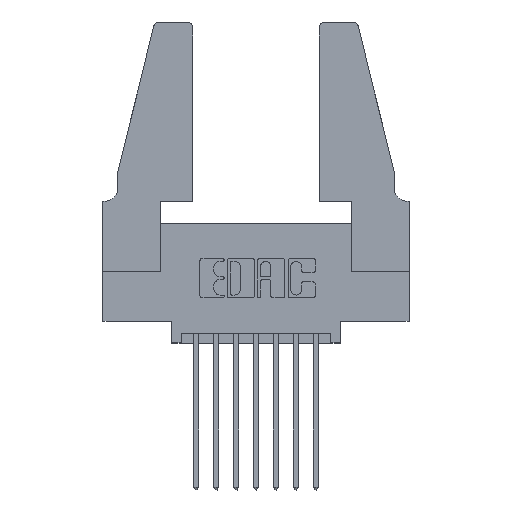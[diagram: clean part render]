
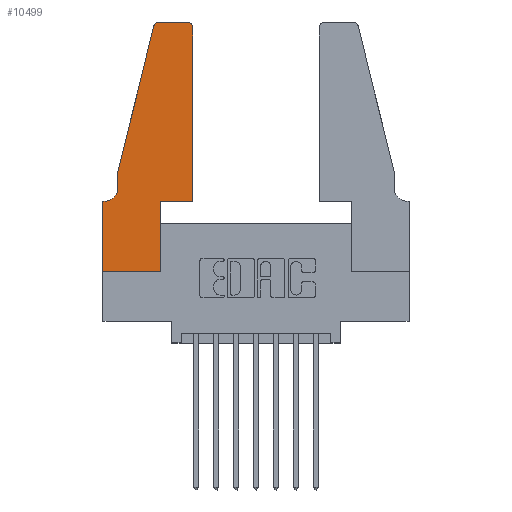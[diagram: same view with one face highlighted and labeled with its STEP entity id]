
A CAD part, top view. The second image highlights one B-rep face of the part: STEP entity #10499.
In plain terms, the highlighted planar face has unit normal (0, 0, 1).
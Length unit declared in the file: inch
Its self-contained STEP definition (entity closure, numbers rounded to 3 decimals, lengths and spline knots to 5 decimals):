
#283 = DIRECTION ( 'NONE',  ( 1., 0., 0. ) ) ;
#386 = CARTESIAN_POINT ( 'NONE',  ( 0.4205, 1.22, 0.37 ) ) ;
#557 = VERTEX_POINT ( 'NONE', #5995 ) ;
#564 = CARTESIAN_POINT ( 'NONE',  ( 0., 0.35, 0.37 ) ) ;
#740 = DIRECTION ( 'NONE',  ( -0.239, -0.971, 0. ) ) ;
#780 = EDGE_CURVE ( 'NONE', #5833, #9450, #3684, .T. ) ;
#1118 = EDGE_CURVE ( 'NONE', #8382, #10596, #7725, .T. ) ;
#1128 = VERTEX_POINT ( 'NONE', #7410 ) ;
#1290 = CARTESIAN_POINT ( 'NONE',  ( 0.4505, 0.35, 0.37 ) ) ;
#1316 = LINE ( 'NONE', #11983, #10981 ) ;
#1511 = VERTEX_POINT ( 'NONE', #10878 ) ;
#1792 = ORIENTED_EDGE ( 'NONE', *, *, #2572, .T. ) ;
#2048 = DIRECTION ( 'NONE',  ( 0., 0., 1. ) ) ;
#2094 = EDGE_CURVE ( 'NONE', #8657, #8382, #12445, .T. ) ;
#2172 = CARTESIAN_POINT ( 'NONE',  ( 0.4505, 1.22, 0.37 ) ) ;
#2437 = CARTESIAN_POINT ( 'NONE',  ( 0.284, 1.25, 0.37 ) ) ;
#2551 = CARTESIAN_POINT ( 'NONE',  ( 0.25487, 1.22718, 0.37 ) ) ;
#2572 = EDGE_CURVE ( 'NONE', #1128, #4253, #7691, .T. ) ;
#2585 = VECTOR ( 'NONE', #8490, 39.37008 ) ;
#2912 = EDGE_CURVE ( 'NONE', #3443, #557, #9167, .T. ) ;
#3052 = VECTOR ( 'NONE', #7720, 39.37008 ) ;
#3119 = LINE ( 'NONE', #10942, #9858 ) ;
#3283 = ORIENTED_EDGE ( 'NONE', *, *, #2094, .T. ) ;
#3354 = DIRECTION ( 'NONE',  ( 0., 1., 0. ) ) ;
#3443 = VERTEX_POINT ( 'NONE', #2551 ) ;
#3461 = VERTEX_POINT ( 'NONE', #7406 ) ;
#3468 = DIRECTION ( 'NONE',  ( -1., 0., 0. ) ) ;
#3496 = DIRECTION ( 'NONE',  ( 0., -1., 0. ) ) ;
#3539 = AXIS2_PLACEMENT_3D ( 'NONE', #11861, #6159, #283 ) ;
#3684 = LINE ( 'NONE', #1290, #10967 ) ;
#3705 = CARTESIAN_POINT ( 'NONE',  ( 0.2865, 0., 0.37 ) ) ;
#3711 = CARTESIAN_POINT ( 'NONE',  ( 0.4205, 1.25, 0.37 ) ) ;
#3883 = DIRECTION ( 'NONE',  ( 0., 0., 1. ) ) ;
#4100 = EDGE_CURVE ( 'NONE', #557, #1511, #11184, .T. ) ;
#4253 = VERTEX_POINT ( 'NONE', #3705 ) ;
#4324 = CIRCLE ( 'NONE', #10275, 0.03 ) ;
#4337 = DIRECTION ( 'NONE',  ( 1., 0., 0. ) ) ;
#4678 = CARTESIAN_POINT ( 'NONE',  ( 0., 0., 0.37 ) ) ;
#4698 = CARTESIAN_POINT ( 'NONE',  ( 0.0755, 0.5, 0.37 ) ) ;
#4815 = DIRECTION ( 'NONE',  ( 0., 0., -1. ) ) ;
#4820 = CARTESIAN_POINT ( 'NONE',  ( 0.2865, 0.35, 0.37 ) ) ;
#5021 = ORIENTED_EDGE ( 'NONE', *, *, #2912, .T. ) ;
#5496 = EDGE_CURVE ( 'NONE', #1511, #3461, #9547, .T. ) ;
#5619 = ORIENTED_EDGE ( 'NONE', *, *, #4100, .T. ) ;
#5741 = AXIS2_PLACEMENT_3D ( 'NONE', #10524, #4815, #11450 ) ;
#5833 = VERTEX_POINT ( 'NONE', #4820 ) ;
#5973 = FACE_OUTER_BOUND ( 'NONE', #11361, .T. ) ;
#5995 = CARTESIAN_POINT ( 'NONE',  ( 0.0755, 0.5, 0.37 ) ) ;
#6159 = DIRECTION ( 'NONE',  ( 0., 0., 1. ) ) ;
#6622 = VECTOR ( 'NONE', #740, 39.37008 ) ;
#6748 = CARTESIAN_POINT ( 'NONE',  ( 0.4505, 0.35, 0.37 ) ) ;
#6868 = EDGE_CURVE ( 'NONE', #11297, #1128, #1316, .T. ) ;
#7126 = ORIENTED_EDGE ( 'NONE', *, *, #5496, .T. ) ;
#7174 = EDGE_CURVE ( 'NONE', #9450, #8657, #10686, .T. ) ;
#7222 = DIRECTION ( 'NONE',  ( 0., -1., 0. ) ) ;
#7270 = ORIENTED_EDGE ( 'NONE', *, *, #11935, .T. ) ;
#7282 = ORIENTED_EDGE ( 'NONE', *, *, #780, .T. ) ;
#7406 = CARTESIAN_POINT ( 'NONE',  ( 0.0055, 0.35, 0.37 ) ) ;
#7410 = CARTESIAN_POINT ( 'NONE',  ( 0., 0., 0.37 ) ) ;
#7424 = ORIENTED_EDGE ( 'NONE', *, *, #9498, .T. ) ;
#7691 = LINE ( 'NONE', #4678, #12435 ) ;
#7720 = DIRECTION ( 'NONE',  ( 0., 1., 0. ) ) ;
#7725 = LINE ( 'NONE', #8121, #2585 ) ;
#7881 = ORIENTED_EDGE ( 'NONE', *, *, #7174, .T. ) ;
#8121 = CARTESIAN_POINT ( 'NONE',  ( 0.2605, 1.25, 0.37 ) ) ;
#8254 = CARTESIAN_POINT ( 'NONE',  ( 0.0755, 0.5, 0.37 ) ) ;
#8382 = VERTEX_POINT ( 'NONE', #3711 ) ;
#8490 = DIRECTION ( 'NONE',  ( -1., 0., 0. ) ) ;
#8633 = DIRECTION ( 'NONE',  ( 1., 0., 0. ) ) ;
#8638 = ORIENTED_EDGE ( 'NONE', *, *, #6868, .T. ) ;
#8657 = VERTEX_POINT ( 'NONE', #2172 ) ;
#8713 = VECTOR ( 'NONE', #3496, 39.37008 ) ;
#9127 = CARTESIAN_POINT ( 'NONE',  ( 0.4505, 0.35, 0.37 ) ) ;
#9167 = LINE ( 'NONE', #4698, #6622 ) ;
#9450 = VERTEX_POINT ( 'NONE', #9127 ) ;
#9451 = VECTOR ( 'NONE', #3468, 39.37008 ) ;
#9498 = EDGE_CURVE ( 'NONE', #3461, #11297, #11956, .T. ) ;
#9501 = ORIENTED_EDGE ( 'NONE', *, *, #1118, .T. ) ;
#9513 = ORIENTED_EDGE ( 'NONE', *, *, #10533, .T. ) ;
#9547 = CIRCLE ( 'NONE', #5741, 0.07 ) ;
#9597 = CARTESIAN_POINT ( 'NONE',  ( 0.284, 1.22, 0.37 ) ) ;
#9858 = VECTOR ( 'NONE', #3354, 39.37008 ) ;
#9888 = DIRECTION ( 'NONE',  ( 1., 0., 0. ) ) ;
#9966 = PLANE ( 'NONE',  #3539 ) ;
#10055 = AXIS2_PLACEMENT_3D ( 'NONE', #386, #2048, #9888 ) ;
#10154 = CARTESIAN_POINT ( 'NONE',  ( 0.0755, 0.35, 0.37 ) ) ;
#10275 = AXIS2_PLACEMENT_3D ( 'NONE', #9597, #3883, #10556 ) ;
#10499 = ADVANCED_FACE ( 'NONE', ( #5973 ), #9966, .T. ) ;
#10524 = CARTESIAN_POINT ( 'NONE',  ( 0.0055, 0.42, 0.37 ) ) ;
#10533 = EDGE_CURVE ( 'NONE', #4253, #5833, #3119, .T. ) ;
#10556 = DIRECTION ( 'NONE',  ( 1., 0., 0. ) ) ;
#10596 = VERTEX_POINT ( 'NONE', #2437 ) ;
#10686 = LINE ( 'NONE', #6748, #3052 ) ;
#10878 = CARTESIAN_POINT ( 'NONE',  ( 0.0755, 0.42, 0.37 ) ) ;
#10942 = CARTESIAN_POINT ( 'NONE',  ( 0.2865, 0.35, 0.37 ) ) ;
#10967 = VECTOR ( 'NONE', #8633, 39.37008 ) ;
#10981 = VECTOR ( 'NONE', #7222, 39.37008 ) ;
#11184 = LINE ( 'NONE', #8254, #8713 ) ;
#11297 = VERTEX_POINT ( 'NONE', #564 ) ;
#11361 = EDGE_LOOP ( 'NONE', ( #9501, #7270, #5021, #5619, #7126, #7424, #8638, #1792, #9513, #7282, #7881, #3283 ) ) ;
#11450 = DIRECTION ( 'NONE',  ( -1., 0., 0. ) ) ;
#11861 = CARTESIAN_POINT ( 'NONE',  ( 0., 0.35, 0.37 ) ) ;
#11935 = EDGE_CURVE ( 'NONE', #10596, #3443, #4324, .T. ) ;
#11956 = LINE ( 'NONE', #10154, #9451 ) ;
#11983 = CARTESIAN_POINT ( 'NONE',  ( 0., 0., 0.37 ) ) ;
#12435 = VECTOR ( 'NONE', #4337, 39.37008 ) ;
#12445 = CIRCLE ( 'NONE', #10055, 0.03 ) ;
